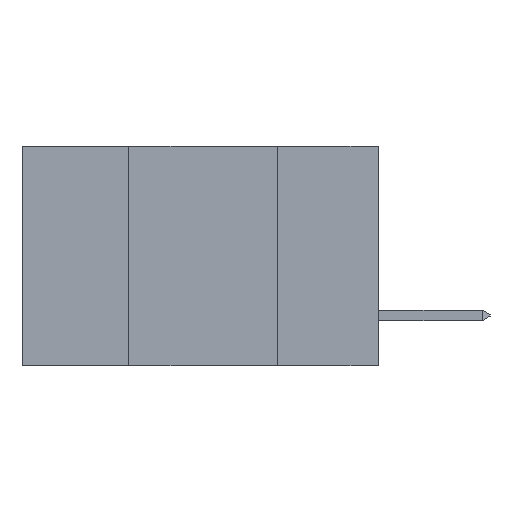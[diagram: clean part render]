
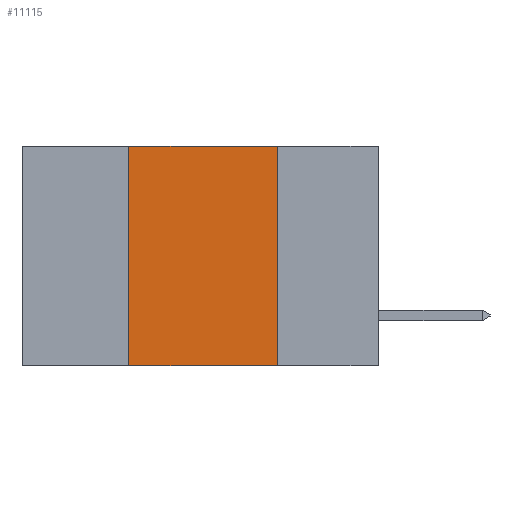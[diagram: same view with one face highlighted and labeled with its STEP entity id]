
A CAD part, left-side view. The second image highlights one B-rep face of the part: STEP entity #11115.
In plain terms, the highlighted planar face has unit normal (-1, 0, 0).
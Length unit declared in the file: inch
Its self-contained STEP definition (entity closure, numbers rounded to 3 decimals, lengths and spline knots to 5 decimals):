
#406 = CARTESIAN_POINT ( 'NONE',  ( 0., 0.6, -0.37 ) ) ;
#463 = CARTESIAN_POINT ( 'NONE',  ( 0., 0.42, 0. ) ) ;
#573 = DIRECTION ( 'NONE',  ( 0., 0., -1. ) ) ;
#1081 = VECTOR ( 'NONE', #13850, 39.37008 ) ;
#1169 = AXIS2_PLACEMENT_3D ( 'NONE', #15482, #8309, #573 ) ;
#1238 = CARTESIAN_POINT ( 'NONE',  ( 0., 0.6, 0. ) ) ;
#1702 = DIRECTION ( 'NONE',  ( 0., -1., 0. ) ) ;
#2522 = ORIENTED_EDGE ( 'NONE', *, *, #9122, .F. ) ;
#3834 = CARTESIAN_POINT ( 'NONE',  ( 0., 0.42, 0. ) ) ;
#3856 = VECTOR ( 'NONE', #1702, 39.37008 ) ;
#4548 = CARTESIAN_POINT ( 'NONE',  ( 0., 0.17, -0.37 ) ) ;
#7524 = CARTESIAN_POINT ( 'NONE',  ( 0., 0.17, 0. ) ) ;
#7764 = CARTESIAN_POINT ( 'NONE',  ( 0., 0.42, -0.37 ) ) ;
#8309 = DIRECTION ( 'NONE',  ( 1., 0., 0. ) ) ;
#8749 = EDGE_CURVE ( 'NONE', #9692, #12437, #12972, .T. ) ;
#9122 = EDGE_CURVE ( 'NONE', #12437, #10071, #14405, .T. ) ;
#9692 = VERTEX_POINT ( 'NONE', #7764 ) ;
#9741 = VECTOR ( 'NONE', #11938, 39.37008 ) ;
#9756 = ORIENTED_EDGE ( 'NONE', *, *, #8749, .F. ) ;
#10022 = VERTEX_POINT ( 'NONE', #4548 ) ;
#10071 = VERTEX_POINT ( 'NONE', #7524 ) ;
#10487 = CARTESIAN_POINT ( 'NONE',  ( 0., 0.17, 0. ) ) ;
#10654 = LINE ( 'NONE', #406, #3856 ) ;
#11043 = EDGE_CURVE ( 'NONE', #9692, #10022, #10654, .T. ) ;
#11115 = ADVANCED_FACE ( 'NONE', ( #15423 ), #14294, .F. ) ;
#11216 = VECTOR ( 'NONE', #11712, 39.37008 ) ;
#11601 = EDGE_CURVE ( 'NONE', #10071, #10022, #14353, .T. ) ;
#11712 = DIRECTION ( 'NONE',  ( 0., 0., -1. ) ) ;
#11938 = DIRECTION ( 'NONE',  ( 0., 0., 1. ) ) ;
#12437 = VERTEX_POINT ( 'NONE', #3834 ) ;
#12972 = LINE ( 'NONE', #463, #9741 ) ;
#13850 = DIRECTION ( 'NONE',  ( 0., -1., 0. ) ) ;
#14294 = PLANE ( 'NONE',  #1169 ) ;
#14353 = LINE ( 'NONE', #10487, #11216 ) ;
#14405 = LINE ( 'NONE', #1238, #1081 ) ;
#14883 = EDGE_LOOP ( 'NONE', ( #15317, #2522, #9756, #16032 ) ) ;
#15317 = ORIENTED_EDGE ( 'NONE', *, *, #11601, .F. ) ;
#15423 = FACE_OUTER_BOUND ( 'NONE', #14883, .T. ) ;
#15482 = CARTESIAN_POINT ( 'NONE',  ( 0., 0.6, 0. ) ) ;
#16032 = ORIENTED_EDGE ( 'NONE', *, *, #11043, .T. ) ;
